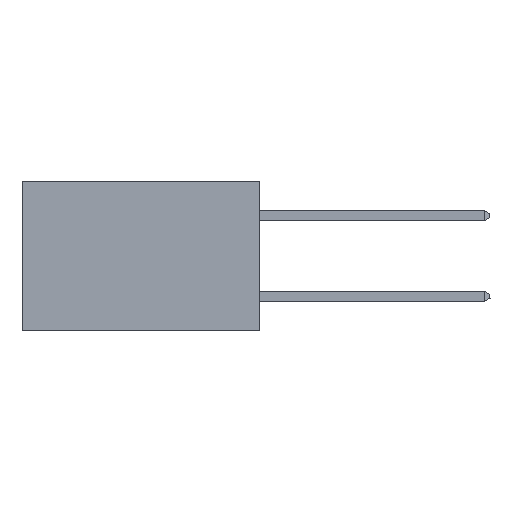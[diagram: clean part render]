
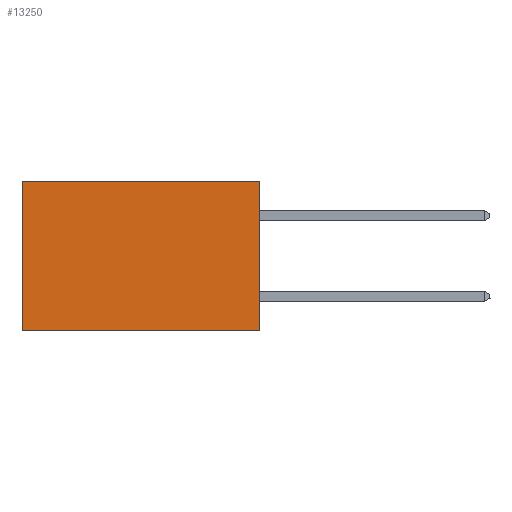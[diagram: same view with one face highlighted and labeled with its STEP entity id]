
A CAD part, left-side view. The second image highlights one B-rep face of the part: STEP entity #13250.
In plain terms, the highlighted planar face has unit normal (-1, 0, 0).
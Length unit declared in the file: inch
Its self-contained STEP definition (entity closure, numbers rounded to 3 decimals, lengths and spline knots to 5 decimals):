
#816 = ORIENTED_EDGE ( 'NONE', *, *, #7264, .F. ) ;
#1623 = CARTESIAN_POINT ( 'NONE',  ( 0.277, 0., 0. ) ) ;
#2132 = ORIENTED_EDGE ( 'NONE', *, *, #19241, .T. ) ;
#2404 = PLANE ( 'NONE',  #4140 ) ;
#2837 = DIRECTION ( 'NONE',  ( 0., 1., 0. ) ) ;
#3575 = VECTOR ( 'NONE', #2837, 39.37008 ) ;
#3947 = ORIENTED_EDGE ( 'NONE', *, *, #7587, .F. ) ;
#4085 = DIRECTION ( 'NONE',  ( 0., 1., 0. ) ) ;
#4140 = AXIS2_PLACEMENT_3D ( 'NONE', #18323, #7409, #18379 ) ;
#4231 = CARTESIAN_POINT ( 'NONE',  ( 0.277, 0., -0.37 ) ) ;
#5114 = VERTEX_POINT ( 'NONE', #10080 ) ;
#7035 = CARTESIAN_POINT ( 'NONE',  ( 0.277, 0., -0.37 ) ) ;
#7068 = EDGE_CURVE ( 'NONE', #18219, #5114, #8276, .T. ) ;
#7144 = VERTEX_POINT ( 'NONE', #7035 ) ;
#7264 = EDGE_CURVE ( 'NONE', #7144, #5114, #12247, .T. ) ;
#7409 = DIRECTION ( 'NONE',  ( 1., 0., 0. ) ) ;
#7587 = EDGE_CURVE ( 'NONE', #8286, #7144, #17377, .T. ) ;
#8011 = VECTOR ( 'NONE', #4085, 39.37008 ) ;
#8276 = LINE ( 'NONE', #17232, #20167 ) ;
#8286 = VERTEX_POINT ( 'NONE', #1623 ) ;
#9986 = CARTESIAN_POINT ( 'NONE',  ( 0.277, 0.59, 0. ) ) ;
#10080 = CARTESIAN_POINT ( 'NONE',  ( 0.277, 0.59, -0.37 ) ) ;
#12247 = LINE ( 'NONE', #4231, #8011 ) ;
#12772 = FACE_OUTER_BOUND ( 'NONE', #15521, .T. ) ;
#13234 = VECTOR ( 'NONE', #13829, 39.37008 ) ;
#13250 = ADVANCED_FACE ( 'NONE', ( #12772 ), #2404, .F. ) ;
#13829 = DIRECTION ( 'NONE',  ( 0., 0., -1. ) ) ;
#14288 = CARTESIAN_POINT ( 'NONE',  ( 0.277, 0., -0.37 ) ) ;
#15521 = EDGE_LOOP ( 'NONE', ( #18986, #816, #3947, #2132 ) ) ;
#15714 = CARTESIAN_POINT ( 'NONE',  ( 0.277, 0., 0. ) ) ;
#17232 = CARTESIAN_POINT ( 'NONE',  ( 0.277, 0.59, -0.37 ) ) ;
#17377 = LINE ( 'NONE', #14288, #13234 ) ;
#17415 = DIRECTION ( 'NONE',  ( 0., 0., -1. ) ) ;
#18219 = VERTEX_POINT ( 'NONE', #9986 ) ;
#18323 = CARTESIAN_POINT ( 'NONE',  ( 0.277, 0., -0.37 ) ) ;
#18379 = DIRECTION ( 'NONE',  ( 0., 0., -1. ) ) ;
#18986 = ORIENTED_EDGE ( 'NONE', *, *, #7068, .T. ) ;
#19241 = EDGE_CURVE ( 'NONE', #8286, #18219, #19829, .T. ) ;
#19829 = LINE ( 'NONE', #15714, #3575 ) ;
#20167 = VECTOR ( 'NONE', #17415, 39.37008 ) ;
